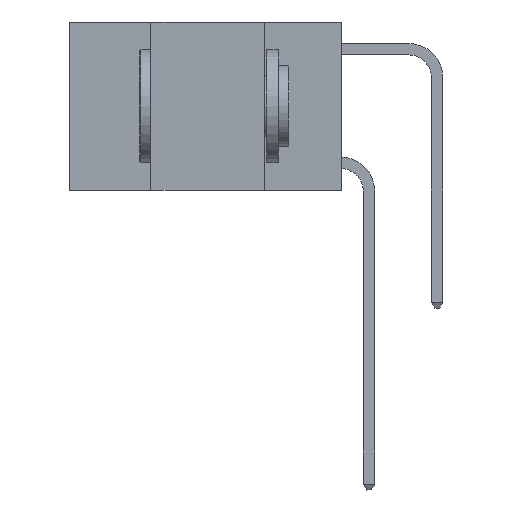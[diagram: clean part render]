
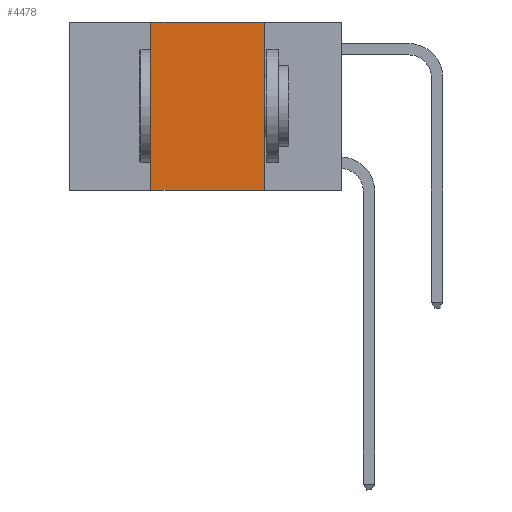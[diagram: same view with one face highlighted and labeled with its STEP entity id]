
A CAD part, left-side view. The second image highlights one B-rep face of the part: STEP entity #4478.
In plain terms, the highlighted planar face has unit normal (-1, 0, 0).
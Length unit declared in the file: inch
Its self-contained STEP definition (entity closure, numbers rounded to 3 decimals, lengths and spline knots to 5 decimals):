
#1028 = LINE ( 'NONE', #7707, #1436 ) ;
#1436 = VECTOR ( 'NONE', #9132, 39.37008 ) ;
#1793 = LINE ( 'NONE', #18443, #8330 ) ;
#2128 = ORIENTED_EDGE ( 'NONE', *, *, #17195, .F. ) ;
#2813 = CARTESIAN_POINT ( 'NONE',  ( 0., 0.6, -0.37 ) ) ;
#3150 = VECTOR ( 'NONE', #18540, 39.37008 ) ;
#3742 = PLANE ( 'NONE',  #19828 ) ;
#4478 = ADVANCED_FACE ( 'NONE', ( #18940 ), #3742, .F. ) ;
#5092 = ORIENTED_EDGE ( 'NONE', *, *, #21106, .F. ) ;
#6448 = CARTESIAN_POINT ( 'NONE',  ( 0., 0.17, 0. ) ) ;
#7707 = CARTESIAN_POINT ( 'NONE',  ( 0., 0.17, 0. ) ) ;
#8221 = VERTEX_POINT ( 'NONE', #17896 ) ;
#8330 = VECTOR ( 'NONE', #13497, 39.37008 ) ;
#8668 = DIRECTION ( 'NONE',  ( 1., 0., 0. ) ) ;
#9132 = DIRECTION ( 'NONE',  ( 0., 0., -1. ) ) ;
#9713 = ORIENTED_EDGE ( 'NONE', *, *, #17872, .T. ) ;
#10612 = CARTESIAN_POINT ( 'NONE',  ( 0., 0.6, 0. ) ) ;
#10724 = VERTEX_POINT ( 'NONE', #6448 ) ;
#13497 = DIRECTION ( 'NONE',  ( 0., -1., 0. ) ) ;
#13967 = CARTESIAN_POINT ( 'NONE',  ( 0., 0.42, 0. ) ) ;
#14010 = DIRECTION ( 'NONE',  ( 0., 0., -1. ) ) ;
#15578 = EDGE_LOOP ( 'NONE', ( #5092, #2128, #18177, #9713 ) ) ;
#16171 = DIRECTION ( 'NONE',  ( 0., -1., 0. ) ) ;
#16190 = CARTESIAN_POINT ( 'NONE',  ( 0., 0.42, -0.37 ) ) ;
#16278 = VERTEX_POINT ( 'NONE', #16190 ) ;
#16568 = LINE ( 'NONE', #20373, #3150 ) ;
#17090 = VECTOR ( 'NONE', #16171, 39.37008 ) ;
#17195 = EDGE_CURVE ( 'NONE', #19293, #10724, #1793, .T. ) ;
#17820 = LINE ( 'NONE', #2813, #17090 ) ;
#17872 = EDGE_CURVE ( 'NONE', #16278, #8221, #17820, .T. ) ;
#17896 = CARTESIAN_POINT ( 'NONE',  ( 0., 0.17, -0.37 ) ) ;
#18177 = ORIENTED_EDGE ( 'NONE', *, *, #20087, .F. ) ;
#18443 = CARTESIAN_POINT ( 'NONE',  ( 0., 0.6, 0. ) ) ;
#18540 = DIRECTION ( 'NONE',  ( 0., 0., 1. ) ) ;
#18940 = FACE_OUTER_BOUND ( 'NONE', #15578, .T. ) ;
#19293 = VERTEX_POINT ( 'NONE', #13967 ) ;
#19828 = AXIS2_PLACEMENT_3D ( 'NONE', #10612, #8668, #14010 ) ;
#20087 = EDGE_CURVE ( 'NONE', #16278, #19293, #16568, .T. ) ;
#20373 = CARTESIAN_POINT ( 'NONE',  ( 0., 0.42, 0. ) ) ;
#21106 = EDGE_CURVE ( 'NONE', #10724, #8221, #1028, .T. ) ;
